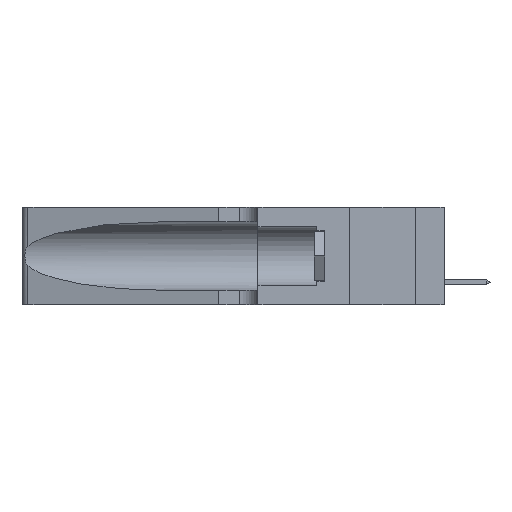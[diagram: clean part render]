
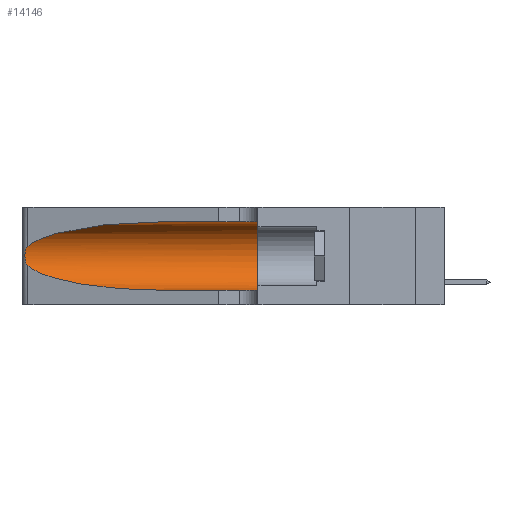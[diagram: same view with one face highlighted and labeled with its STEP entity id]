
A CAD part, left-side view. The second image highlights one B-rep face of the part: STEP entity #14146.
In plain terms, the highlighted cylindrical face has radius 3.308 mm (diameter 6.617 mm), a partial arc.
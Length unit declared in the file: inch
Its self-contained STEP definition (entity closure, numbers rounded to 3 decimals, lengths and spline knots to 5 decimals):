
#186 = VERTEX_POINT ( 'NONE', #2094 ) ;
#1196 = DIRECTION ( 'NONE',  ( 0., -1., 0. ) ) ;
#2094 = CARTESIAN_POINT ( 'NONE',  ( 0.25487, 1.22718, 0.14631 ) ) ;
#2863 = CARTESIAN_POINT ( 'NONE',  ( 0.25487, 1.22718, 0.22369 ) ) ;
#3277 = EDGE_CURVE ( 'NONE', #6485, #186, #36933, .T. ) ;
#3519 = CARTESIAN_POINT ( 'NONE',  ( 0.25639, 1.23186, 0.15144 ) ) ;
#4354 = CARTESIAN_POINT ( 'NONE',  ( 0.25487, 1.22718, 0.14631 ) ) ;
#5320 = ORIENTED_EDGE ( 'NONE', *, *, #3277, .T. ) ;
#6485 = VERTEX_POINT ( 'NONE', #8985 ) ;
#6682 = DIRECTION ( 'NONE',  ( 0., -1., 0. ) ) ;
#6916 = CARTESIAN_POINT ( 'NONE',  ( 0.26018, 1.23835, 0.19895 ) ) ;
#7398 = CARTESIAN_POINT ( 'NONE',  ( 0.25789, 1.23486, 0.15765 ) ) ;
#8985 = CARTESIAN_POINT ( 'NONE',  ( 0.25487, 1.22718, 0.22369 ) ) ;
#9550 = DIRECTION ( 'NONE',  ( 0., 0., 1. ) ) ;
#10161 = CARTESIAN_POINT ( 'NONE',  ( 0.18966, 0.96281, 0.31525 ) ) ;
#10937 = VECTOR ( 'NONE', #6682, 39.37008 ) ;
#11103 = CARTESIAN_POINT ( 'NONE',  ( 0.26075, 1.23896, 0.19203 ) ) ;
#11772 = VERTEX_POINT ( 'NONE', #16078 ) ;
#12715 = CARTESIAN_POINT ( 'NONE',  ( 0.1305, 1.61858, 0.05475 ) ) ;
#14146 = ADVANCED_FACE ( 'NONE', ( #37986 ), #33925, .F. ) ;
#14531 = CARTESIAN_POINT ( 'NONE',  ( 0.25787, 1.23484, 0.2124 ) ) ;
#14862 = CARTESIAN_POINT ( 'NONE',  ( 0.25487, 1.22718, 0.14631 ) ) ;
#14939 = EDGE_CURVE ( 'NONE', #22996, #19169, #37898, .T. ) ;
#15277 = EDGE_CURVE ( 'NONE', #11772, #6485, #30570, .T. ) ;
#16078 = CARTESIAN_POINT ( 'NONE',  ( 0.1305, 0.72297, 0.31525 ) ) ;
#16765 = LINE ( 'NONE', #12715, #40201 ) ;
#17235 = CARTESIAN_POINT ( 'NONE',  ( 0.1305, 1.61858, 0.31525 ) ) ;
#17323 = CARTESIAN_POINT ( 'NONE',  ( 0.2373, 1.15595, 0.28018 ) ) ;
#17948 = CARTESIAN_POINT ( 'NONE',  ( 0.25856, 1.23593, 0.16098 ) ) ;
#18282 = CARTESIAN_POINT ( 'NONE',  ( 0.26075, 1.23896, 0.178 ) ) ;
#19169 = VERTEX_POINT ( 'NONE', #21618 ) ;
#19494 = ORIENTED_EDGE ( 'NONE', *, *, #47140, .F. ) ;
#21264 = ORIENTED_EDGE ( 'NONE', *, *, #26630, .T. ) ;
#21618 = CARTESIAN_POINT ( 'NONE',  ( 0.1305, 0.35, 0.05475 ) ) ;
#22068 = LINE ( 'NONE', #17235, #10937 ) ;
#22996 = VERTEX_POINT ( 'NONE', #41399 ) ;
#23383 = CARTESIAN_POINT ( 'NONE',  ( 0.2373, 1.15595, 0.08982 ) ) ;
#24509 = CARTESIAN_POINT ( 'NONE',  ( 0.25555, 1.22993, 0.14849 ) ) ;
#25006 = CARTESIAN_POINT ( 'NONE',  ( 0.1305, 0.72297, 0.05475 ) ) ;
#25477 = CARTESIAN_POINT ( 'NONE',  ( 0.25639, 1.23184, 0.21858 ) ) ;
#26630 = EDGE_CURVE ( 'NONE', #186, #43835, #31173, .T. ) ;
#27137 = CARTESIAN_POINT ( 'NONE',  ( 0.1305, 0.72297, 0.05475 ) ) ;
#27847 = EDGE_CURVE ( 'NONE', #43835, #19169, #16765, .T. ) ;
#28633 = DIRECTION ( 'NONE',  ( 0., 1., 0. ) ) ;
#29068 = CARTESIAN_POINT ( 'NONE',  ( 0.1305, 0.72297, 0.31525 ) ) ;
#30570 =( BOUNDED_CURVE ( )  B_SPLINE_CURVE ( 3, ( #29068, #10161, #17323, #2863 ),
 .UNSPECIFIED., .F., .T. ) 
 B_SPLINE_CURVE_WITH_KNOTS ( ( 4, 4 ),
 ( 1.5708, 2.84003 ),
 .UNSPECIFIED. ) 
 CURVE ( )  GEOMETRIC_REPRESENTATION_ITEM ( )  RATIONAL_B_SPLINE_CURVE ( ( 1., 0.87, 0.87, 1. ) ) 
 REPRESENTATION_ITEM ( '' )  );
#31173 =( BOUNDED_CURVE ( )  B_SPLINE_CURVE ( 3, ( #4354, #23383, #36136, #25006 ),
 .UNSPECIFIED., .F., .F. ) 
 B_SPLINE_CURVE_WITH_KNOTS ( ( 4, 4 ),
 ( 3.44316, 4.71239 ),
 .UNSPECIFIED. ) 
 CURVE ( )  GEOMETRIC_REPRESENTATION_ITEM ( )  RATIONAL_B_SPLINE_CURVE ( ( 1., 0.87, 0.87, 1. ) ) 
 REPRESENTATION_ITEM ( '' )  );
#31839 = ORIENTED_EDGE ( 'NONE', *, *, #27847, .T. ) ;
#33013 = CARTESIAN_POINT ( 'NONE',  ( 0.26017, 1.23833, 0.17102 ) ) ;
#33608 = ORIENTED_EDGE ( 'NONE', *, *, #14939, .F. ) ;
#33925 = CYLINDRICAL_SURFACE ( 'NONE', #42056, 0.13025 ) ;
#34764 = DIRECTION ( 'NONE',  ( 0., -1., 0. ) ) ;
#35086 = CARTESIAN_POINT ( 'NONE',  ( 0.1305, 1.61858, 0.185 ) ) ;
#36136 = CARTESIAN_POINT ( 'NONE',  ( 0.18966, 0.96281, 0.05475 ) ) ;
#36333 = CARTESIAN_POINT ( 'NONE',  ( 0.1305, 0.35, 0.185 ) ) ;
#36933 = B_SPLINE_CURVE_WITH_KNOTS ( 'NONE', 3,
 ( #47976, #37107, #25477, #14531, #40523, #6916, #11103, #18282, #33013, #17948, #7398, #3519, #24509, #14862 ),
 .UNSPECIFIED., .F., .F.,
 ( 4, 2, 2, 2, 2, 2, 4 ),
 ( 0., 0.00027, 0.00053, 0.00107, 0.0016, 0.00187, 0.00214 ),
 .UNSPECIFIED. ) ;
#37107 = CARTESIAN_POINT ( 'NONE',  ( 0.25555, 1.22994, 0.2215 ) ) ;
#37898 = CIRCLE ( 'NONE', #38653, 0.13025 ) ;
#37986 = FACE_OUTER_BOUND ( 'NONE', #44926, .T. ) ;
#38050 = ORIENTED_EDGE ( 'NONE', *, *, #15277, .T. ) ;
#38653 = AXIS2_PLACEMENT_3D ( 'NONE', #36333, #28633, #9550 ) ;
#40201 = VECTOR ( 'NONE', #1196, 39.37008 ) ;
#40523 = CARTESIAN_POINT ( 'NONE',  ( 0.25854, 1.2359, 0.20912 ) ) ;
#41399 = CARTESIAN_POINT ( 'NONE',  ( 0.1305, 0.35, 0.31525 ) ) ;
#42056 = AXIS2_PLACEMENT_3D ( 'NONE', #35086, #34764, #45795 ) ;
#43835 = VERTEX_POINT ( 'NONE', #27137 ) ;
#44926 = EDGE_LOOP ( 'NONE', ( #38050, #5320, #21264, #31839, #33608, #19494 ) ) ;
#45795 = DIRECTION ( 'NONE',  ( 0., 0., -1. ) ) ;
#47140 = EDGE_CURVE ( 'NONE', #11772, #22996, #22068, .T. ) ;
#47976 = CARTESIAN_POINT ( 'NONE',  ( 0.25487, 1.22718, 0.22369 ) ) ;
